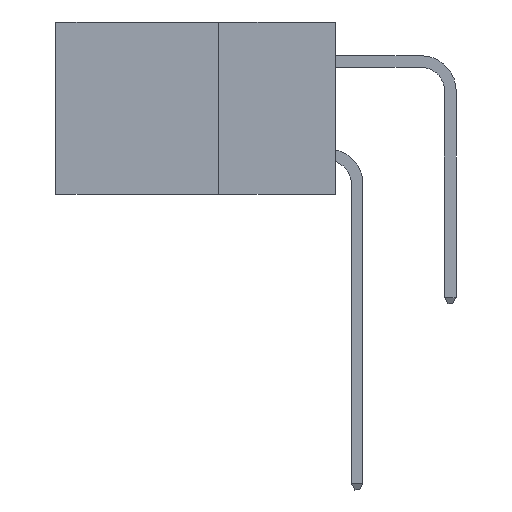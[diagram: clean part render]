
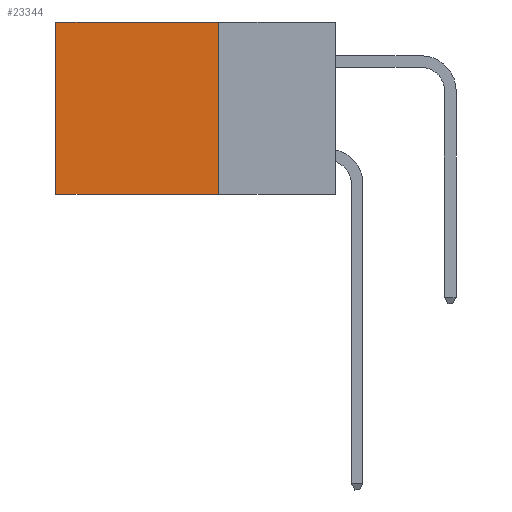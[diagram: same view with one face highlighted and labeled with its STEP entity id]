
A CAD part, left-side view. The second image highlights one B-rep face of the part: STEP entity #23344.
In plain terms, the highlighted planar face has unit normal (-1, 0, 0).
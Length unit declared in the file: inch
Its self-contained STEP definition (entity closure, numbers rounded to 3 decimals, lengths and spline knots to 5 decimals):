
#805 = VECTOR ( 'NONE', #10436, 39.37008 ) ;
#2194 = VERTEX_POINT ( 'NONE', #17547 ) ;
#2318 = VECTOR ( 'NONE', #21951, 39.37008 ) ;
#2395 = VERTEX_POINT ( 'NONE', #16011 ) ;
#2973 = DIRECTION ( 'NONE',  ( 0., 0., -1. ) ) ;
#3221 = EDGE_LOOP ( 'NONE', ( #19406, #15754, #12323, #4449 ) ) ;
#4063 = CARTESIAN_POINT ( 'NONE',  ( 0.2875, 0.25, 0. ) ) ;
#4449 = ORIENTED_EDGE ( 'NONE', *, *, #18764, .T. ) ;
#4502 = LINE ( 'NONE', #21191, #805 ) ;
#5647 = CARTESIAN_POINT ( 'NONE',  ( 0.2875, 0.25, -0.37 ) ) ;
#5979 = EDGE_CURVE ( 'NONE', #2395, #22640, #12421, .T. ) ;
#7901 = VERTEX_POINT ( 'NONE', #20873 ) ;
#8428 = DIRECTION ( 'NONE',  ( 0., 1., 0. ) ) ;
#10436 = DIRECTION ( 'NONE',  ( 0., 0., -1. ) ) ;
#10448 = LINE ( 'NONE', #13766, #11648 ) ;
#11648 = VECTOR ( 'NONE', #8428, 39.37008 ) ;
#12242 = EDGE_CURVE ( 'NONE', #7901, #2395, #15085, .T. ) ;
#12323 = ORIENTED_EDGE ( 'NONE', *, *, #12242, .F. ) ;
#12421 = LINE ( 'NONE', #5647, #21842 ) ;
#13756 = PLANE ( 'NONE',  #15516 ) ;
#13766 = CARTESIAN_POINT ( 'NONE',  ( 0.2875, 0.25, 0. ) ) ;
#15085 = LINE ( 'NONE', #4063, #2318 ) ;
#15516 = AXIS2_PLACEMENT_3D ( 'NONE', #22963, #19187, #2973 ) ;
#15526 = FACE_OUTER_BOUND ( 'NONE', #3221, .T. ) ;
#15754 = ORIENTED_EDGE ( 'NONE', *, *, #5979, .F. ) ;
#16011 = CARTESIAN_POINT ( 'NONE',  ( 0.2875, 0.25, -0.37 ) ) ;
#16392 = CARTESIAN_POINT ( 'NONE',  ( 0.2875, 0.6, -0.37 ) ) ;
#17547 = CARTESIAN_POINT ( 'NONE',  ( 0.2875, 0.6, 0. ) ) ;
#17958 = DIRECTION ( 'NONE',  ( 0., 1., 0. ) ) ;
#18764 = EDGE_CURVE ( 'NONE', #7901, #2194, #10448, .T. ) ;
#19187 = DIRECTION ( 'NONE',  ( 1., 0., 0. ) ) ;
#19406 = ORIENTED_EDGE ( 'NONE', *, *, #23262, .T. ) ;
#20873 = CARTESIAN_POINT ( 'NONE',  ( 0.2875, 0.25, 0. ) ) ;
#21191 = CARTESIAN_POINT ( 'NONE',  ( 0.2875, 0.6, 0. ) ) ;
#21842 = VECTOR ( 'NONE', #17958, 39.37008 ) ;
#21951 = DIRECTION ( 'NONE',  ( 0., 0., -1. ) ) ;
#22640 = VERTEX_POINT ( 'NONE', #16392 ) ;
#22963 = CARTESIAN_POINT ( 'NONE',  ( 0.2875, 0.25, 0. ) ) ;
#23262 = EDGE_CURVE ( 'NONE', #2194, #22640, #4502, .T. ) ;
#23344 = ADVANCED_FACE ( 'NONE', ( #15526 ), #13756, .F. ) ;
